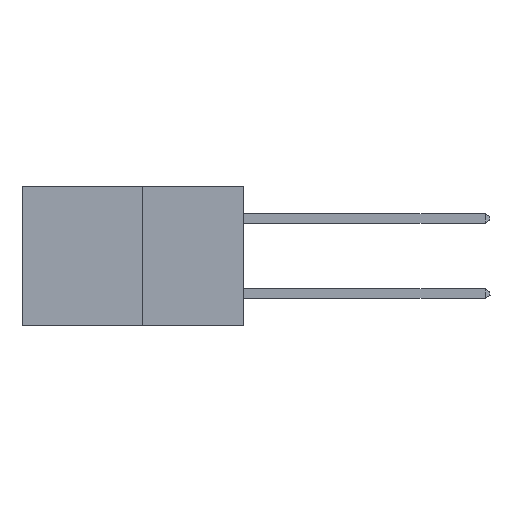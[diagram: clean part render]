
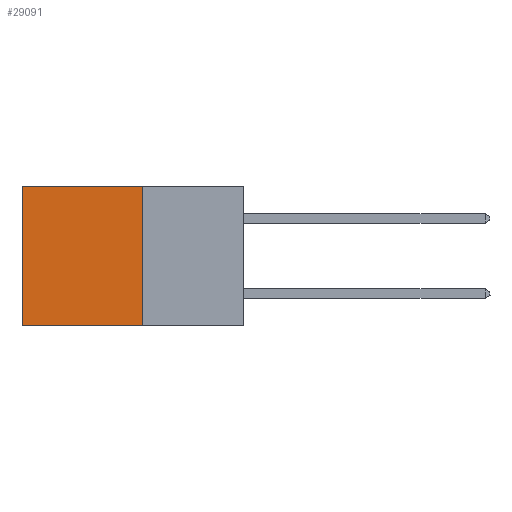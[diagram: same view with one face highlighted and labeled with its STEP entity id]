
A CAD part, left-side view. The second image highlights one B-rep face of the part: STEP entity #29091.
In plain terms, the highlighted planar face has unit normal (-1, 0, 0).
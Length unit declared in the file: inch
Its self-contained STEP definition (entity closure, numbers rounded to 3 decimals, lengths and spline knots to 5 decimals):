
#1083 = EDGE_CURVE ( 'NONE', #21404, #27386, #14624, .T. ) ;
#1571 = DIRECTION ( 'NONE',  ( 0., 1., 0. ) ) ;
#2271 = FACE_OUTER_BOUND ( 'NONE', #23491, .T. ) ;
#2540 = LINE ( 'NONE', #8199, #10098 ) ;
#3491 = DIRECTION ( 'NONE',  ( 0., 1., 0. ) ) ;
#3623 = EDGE_CURVE ( 'NONE', #26027, #5015, #16807, .T. ) ;
#3853 = AXIS2_PLACEMENT_3D ( 'NONE', #25725, #10595, #28353 ) ;
#4090 = ORIENTED_EDGE ( 'NONE', *, *, #1083, .T. ) ;
#4320 = CARTESIAN_POINT ( 'NONE',  ( 0.277, 0.59, -0.37 ) ) ;
#5015 = VERTEX_POINT ( 'NONE', #4320 ) ;
#7463 = CARTESIAN_POINT ( 'NONE',  ( 0.277, 0.27, -0.37 ) ) ;
#8048 = PLANE ( 'NONE',  #3853 ) ;
#8199 = CARTESIAN_POINT ( 'NONE',  ( 0.277, 0.27, -0.37 ) ) ;
#9958 = LINE ( 'NONE', #19911, #22719 ) ;
#9991 = VECTOR ( 'NONE', #1571, 39.37008 ) ;
#10098 = VECTOR ( 'NONE', #28507, 39.37008 ) ;
#10595 = DIRECTION ( 'NONE',  ( 1., 0., 0. ) ) ;
#11695 = ORIENTED_EDGE ( 'NONE', *, *, #3623, .F. ) ;
#14624 = LINE ( 'NONE', #24941, #20563 ) ;
#14654 = EDGE_CURVE ( 'NONE', #27386, #5015, #9958, .T. ) ;
#16807 = LINE ( 'NONE', #7463, #9991 ) ;
#19173 = EDGE_CURVE ( 'NONE', #21404, #26027, #2540, .T. ) ;
#19611 = CARTESIAN_POINT ( 'NONE',  ( 0.277, 0.59, 0. ) ) ;
#19911 = CARTESIAN_POINT ( 'NONE',  ( 0.277, 0.59, -0.37 ) ) ;
#20563 = VECTOR ( 'NONE', #3491, 39.37008 ) ;
#20806 = CARTESIAN_POINT ( 'NONE',  ( 0.277, 0.27, -0.37 ) ) ;
#21404 = VERTEX_POINT ( 'NONE', #23866 ) ;
#22286 = ORIENTED_EDGE ( 'NONE', *, *, #19173, .F. ) ;
#22464 = DIRECTION ( 'NONE',  ( 0., 0., -1. ) ) ;
#22719 = VECTOR ( 'NONE', #22464, 39.37008 ) ;
#23468 = ORIENTED_EDGE ( 'NONE', *, *, #14654, .T. ) ;
#23491 = EDGE_LOOP ( 'NONE', ( #23468, #11695, #22286, #4090 ) ) ;
#23866 = CARTESIAN_POINT ( 'NONE',  ( 0.277, 0.27, 0. ) ) ;
#24941 = CARTESIAN_POINT ( 'NONE',  ( 0.277, 0.27, 0. ) ) ;
#25725 = CARTESIAN_POINT ( 'NONE',  ( 0.277, 0.27, -0.37 ) ) ;
#26027 = VERTEX_POINT ( 'NONE', #20806 ) ;
#27386 = VERTEX_POINT ( 'NONE', #19611 ) ;
#28353 = DIRECTION ( 'NONE',  ( 0., 0., -1. ) ) ;
#28507 = DIRECTION ( 'NONE',  ( 0., 0., -1. ) ) ;
#29091 = ADVANCED_FACE ( 'NONE', ( #2271 ), #8048, .F. ) ;
